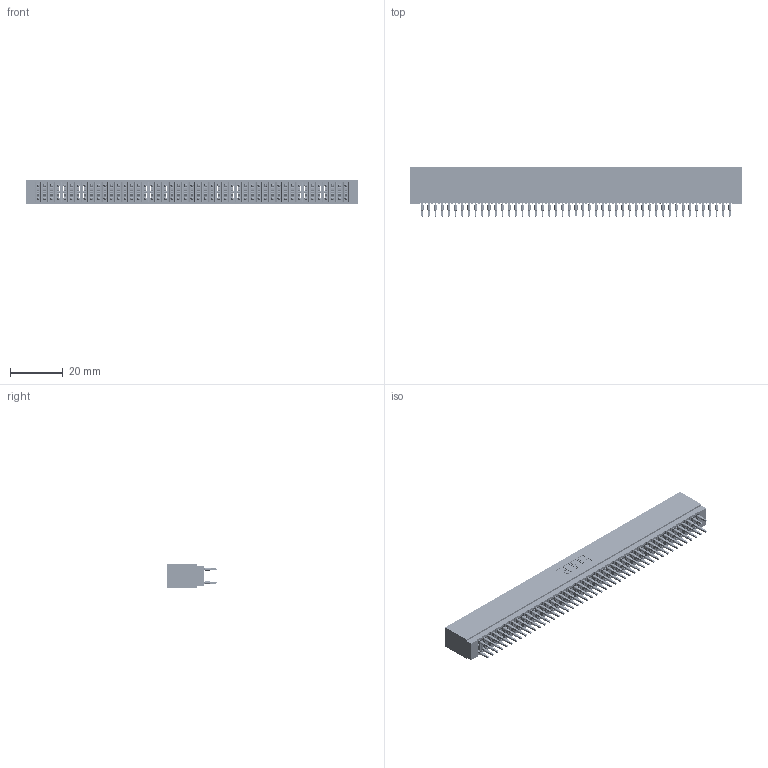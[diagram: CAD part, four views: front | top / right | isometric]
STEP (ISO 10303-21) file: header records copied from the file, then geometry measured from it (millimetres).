
FILE_DESCRIPTION (( 'STEP AP203' ), '1' );
FILE_NAME ('725-094-560-201.STEP', '2026-02-24T19:42:45', ( '' ), ( '' ), 'SwSTEP 2.0', 'SolidWorks 2023', '' );
FILE_SCHEMA (( 'CONFIG_CONTROL_DESIGN' ));
Products named in the file (3): 725 Part_Insulator Option - 01; 745-292-001_560; 725-094-560-201
Assembly tree (95 placements, depth 2):
  725-094-560-201
    725 Part_Insulator Option - 01
    745-292-001_560  x94
Bounding box: 125.98 x 18.8 x 8.89 mm (x, y, z)
Volume: 10312.7 mm3; surface area: 23370.8 mm2
Topology: 95 solids, 95 shells, 9354 faces, 25587 edges, 16242 vertices
Faces by surface type: plane 4849, cylinder 2061, bspline 1880, torus 564
Entity records: 78730 total; most frequent: CARTESIAN_POINT 14157, ORIENTED_EDGE 13602, DIRECTION 11885, EDGE_CURVE 6801, LINE 6329, VECTOR 6329, VERTEX_POINT 4338, AXIS2_PLACEMENT_3D 2778
